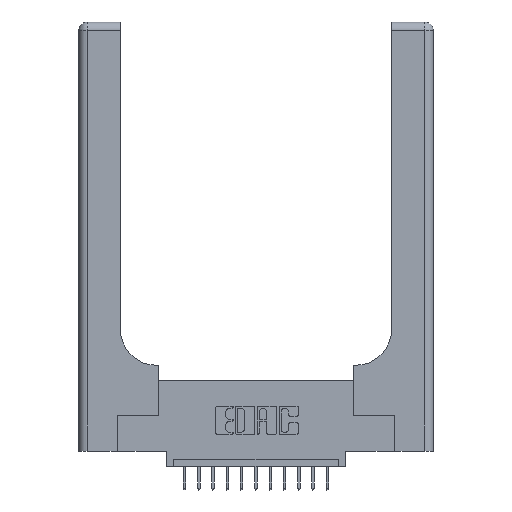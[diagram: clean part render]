
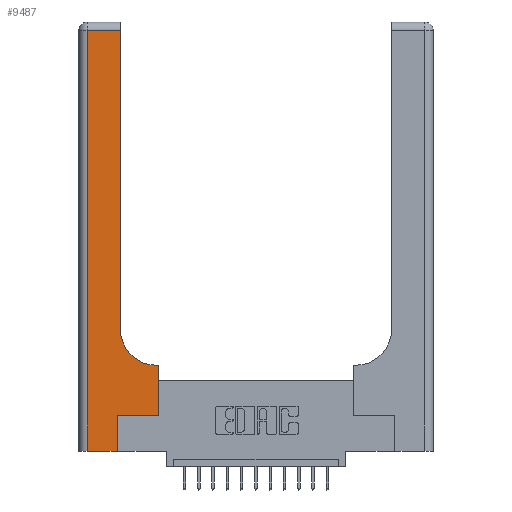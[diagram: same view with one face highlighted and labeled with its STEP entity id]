
A CAD part, top view. The second image highlights one B-rep face of the part: STEP entity #9487.
In plain terms, the highlighted planar face has unit normal (0, 0, 1).
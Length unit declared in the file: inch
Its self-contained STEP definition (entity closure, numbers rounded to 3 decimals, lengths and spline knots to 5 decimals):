
#38 = DIRECTION ( 'NONE',  ( 0., 1., 0. ) ) ;
#222 = DIRECTION ( 'NONE',  ( 1., 0., 0. ) ) ;
#342 = DIRECTION ( 'NONE',  ( 1., 0., 0. ) ) ;
#592 = EDGE_CURVE ( 'NONE', #11262, #4849, #16619, .T. ) ;
#1135 = CARTESIAN_POINT ( 'NONE',  ( 0.06, 0., 0.37 ) ) ;
#1224 = AXIS2_PLACEMENT_3D ( 'NONE', #10347, #11674, #3556 ) ;
#1677 = DIRECTION ( 'NONE',  ( 0., 0., -1. ) ) ;
#1681 = ORIENTED_EDGE ( 'NONE', *, *, #592, .T. ) ;
#2023 = VECTOR ( 'NONE', #12743, 39.37008 ) ;
#2448 = VECTOR ( 'NONE', #8419, 39.37008 ) ;
#3103 = ORIENTED_EDGE ( 'NONE', *, *, #12662, .T. ) ;
#3556 = DIRECTION ( 'NONE',  ( -1., 0., 0. ) ) ;
#3563 = DIRECTION ( 'NONE',  ( 0., -1., 0. ) ) ;
#3714 = VERTEX_POINT ( 'NONE', #11669 ) ;
#3846 = DIRECTION ( 'NONE',  ( 0., 1., 0. ) ) ;
#3972 = AXIS2_PLACEMENT_3D ( 'NONE', #13989, #1677, #342 ) ;
#3995 = ORIENTED_EDGE ( 'NONE', *, *, #7715, .T. ) ;
#4272 = VECTOR ( 'NONE', #38, 39.37008 ) ;
#4707 = LINE ( 'NONE', #13698, #4272 ) ;
#4848 = LINE ( 'NONE', #5157, #13916 ) ;
#4849 = VERTEX_POINT ( 'NONE', #17035 ) ;
#5019 = EDGE_LOOP ( 'NONE', ( #17733, #10819, #3995, #3103, #12927, #15464, #16078, #6280, #1681 ) ) ;
#5065 = LINE ( 'NONE', #7113, #2023 ) ;
#5067 = VERTEX_POINT ( 'NONE', #1135 ) ;
#5157 = CARTESIAN_POINT ( 'NONE',  ( 0., 0., 0.37 ) ) ;
#5492 = LINE ( 'NONE', #11159, #13895 ) ;
#5884 = CARTESIAN_POINT ( 'NONE',  ( 0.06, 2.94, 0.37 ) ) ;
#6280 = ORIENTED_EDGE ( 'NONE', *, *, #8853, .T. ) ;
#6302 = EDGE_CURVE ( 'NONE', #3714, #8173, #4707, .T. ) ;
#6531 = DIRECTION ( 'NONE',  ( 1., 0., 0. ) ) ;
#6723 = CARTESIAN_POINT ( 'NONE',  ( 0.269, 0., 0.37 ) ) ;
#7113 = CARTESIAN_POINT ( 'NONE',  ( 0., 2.94, 0.37 ) ) ;
#7170 = DIRECTION ( 'NONE',  ( 0., 1., 0. ) ) ;
#7715 = EDGE_CURVE ( 'NONE', #12450, #5067, #9211, .T. ) ;
#7813 = CARTESIAN_POINT ( 'NONE',  ( 0.06, 3., 0.37 ) ) ;
#8173 = VERTEX_POINT ( 'NONE', #17804 ) ;
#8419 = DIRECTION ( 'NONE',  ( -1., 0., 0. ) ) ;
#8721 = CARTESIAN_POINT ( 'NONE',  ( 0.269, 0., 0.37 ) ) ;
#8853 = EDGE_CURVE ( 'NONE', #8173, #11262, #9758, .T. ) ;
#9001 = VERTEX_POINT ( 'NONE', #8721 ) ;
#9137 = VERTEX_POINT ( 'NONE', #9258 ) ;
#9211 = LINE ( 'NONE', #7813, #16108 ) ;
#9258 = CARTESIAN_POINT ( 'NONE',  ( 0.2915, 2.94, 0.37 ) ) ;
#9442 = VECTOR ( 'NONE', #222, 39.37008 ) ;
#9487 = ADVANCED_FACE ( 'NONE', ( #12994 ), #17186, .F. ) ;
#9563 = CARTESIAN_POINT ( 'NONE',  ( 0.5415, 0.6, 0.37 ) ) ;
#9758 = LINE ( 'NONE', #13987, #2448 ) ;
#10347 = CARTESIAN_POINT ( 'NONE',  ( 0., 3., 0.37 ) ) ;
#10819 = ORIENTED_EDGE ( 'NONE', *, *, #13079, .T. ) ;
#11159 = CARTESIAN_POINT ( 'NONE',  ( 0.2915, 3., 0.37 ) ) ;
#11262 = VERTEX_POINT ( 'NONE', #9563 ) ;
#11306 = EDGE_CURVE ( 'NONE', #17093, #3714, #15065, .T. ) ;
#11669 = CARTESIAN_POINT ( 'NONE',  ( 0.5585, 0.25, 0.37 ) ) ;
#11674 = DIRECTION ( 'NONE',  ( 0., 0., -1. ) ) ;
#12450 = VERTEX_POINT ( 'NONE', #5884 ) ;
#12662 = EDGE_CURVE ( 'NONE', #5067, #9001, #4848, .T. ) ;
#12743 = DIRECTION ( 'NONE',  ( -1., 0., 0. ) ) ;
#12927 = ORIENTED_EDGE ( 'NONE', *, *, #15160, .T. ) ;
#12994 = FACE_OUTER_BOUND ( 'NONE', #5019, .T. ) ;
#13012 = EDGE_CURVE ( 'NONE', #4849, #9137, #5492, .T. ) ;
#13079 = EDGE_CURVE ( 'NONE', #9137, #12450, #5065, .T. ) ;
#13183 = LINE ( 'NONE', #6723, #15101 ) ;
#13698 = CARTESIAN_POINT ( 'NONE',  ( 0.5585, 0.25, 0.37 ) ) ;
#13895 = VECTOR ( 'NONE', #7170, 39.37008 ) ;
#13916 = VECTOR ( 'NONE', #6531, 39.37008 ) ;
#13987 = CARTESIAN_POINT ( 'NONE',  ( 0.2915, 0.6, 0.37 ) ) ;
#13989 = CARTESIAN_POINT ( 'NONE',  ( 0.5415, 0.85, 0.37 ) ) ;
#15065 = LINE ( 'NONE', #16704, #9442 ) ;
#15101 = VECTOR ( 'NONE', #3846, 39.37008 ) ;
#15160 = EDGE_CURVE ( 'NONE', #9001, #17093, #13183, .T. ) ;
#15432 = CARTESIAN_POINT ( 'NONE',  ( 0.269, 0.25, 0.37 ) ) ;
#15464 = ORIENTED_EDGE ( 'NONE', *, *, #11306, .T. ) ;
#16078 = ORIENTED_EDGE ( 'NONE', *, *, #6302, .T. ) ;
#16108 = VECTOR ( 'NONE', #3563, 39.37008 ) ;
#16619 = CIRCLE ( 'NONE', #3972, 0.25 ) ;
#16704 = CARTESIAN_POINT ( 'NONE',  ( 0.269, 0.25, 0.37 ) ) ;
#17035 = CARTESIAN_POINT ( 'NONE',  ( 0.2915, 0.85, 0.37 ) ) ;
#17093 = VERTEX_POINT ( 'NONE', #15432 ) ;
#17186 = PLANE ( 'NONE',  #1224 ) ;
#17733 = ORIENTED_EDGE ( 'NONE', *, *, #13012, .T. ) ;
#17804 = CARTESIAN_POINT ( 'NONE',  ( 0.5585, 0.6, 0.37 ) ) ;
